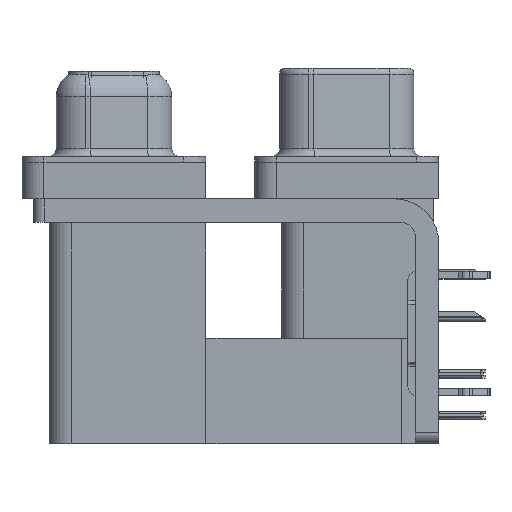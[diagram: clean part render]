
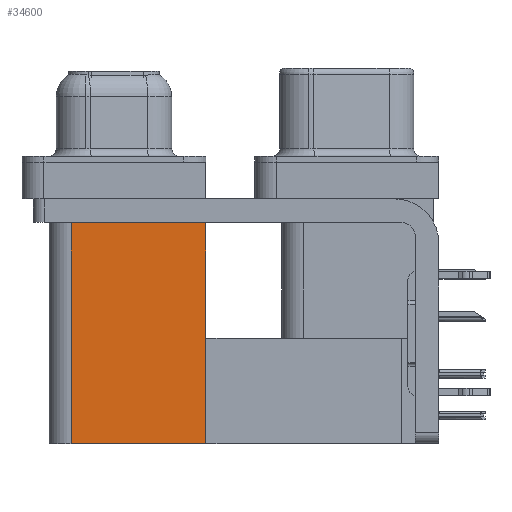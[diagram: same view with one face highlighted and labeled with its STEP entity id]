
A CAD part, left-side view. The second image highlights one B-rep face of the part: STEP entity #34600.
In plain terms, the highlighted planar face has unit normal (-1, 0, 0).
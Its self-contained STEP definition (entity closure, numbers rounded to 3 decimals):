
#1428 = VERTEX_POINT ( 'NONE', #48696 ) ;
#1985 = EDGE_CURVE ( 'NONE', #21055, #7753, #45474, .T. ) ;
#3163 = CARTESIAN_POINT ( 'NONE',  ( 3.7, 18.8, -19.2 ) ) ;
#4700 = VECTOR ( 'NONE', #24613, 1000. ) ;
#5008 = ORIENTED_EDGE ( 'NONE', *, *, #6114, .T. ) ;
#6114 = EDGE_CURVE ( 'NONE', #20795, #1428, #52254, .T. ) ;
#6152 = DIRECTION ( 'NONE',  ( 0., 0., -1. ) ) ;
#7625 = CARTESIAN_POINT ( 'NONE',  ( 3.7, 9.6, -2.5 ) ) ;
#7753 = VERTEX_POINT ( 'NONE', #36050 ) ;
#10634 = EDGE_CURVE ( 'NONE', #1428, #7753, #16259, .T. ) ;
#11768 = CARTESIAN_POINT ( 'NONE',  ( 3.7, 18.8, -19.2 ) ) ;
#14082 = DIRECTION ( 'NONE',  ( 0., 0., 1. ) ) ;
#14524 = PLANE ( 'NONE',  #26805 ) ;
#14706 = CARTESIAN_POINT ( 'NONE',  ( 3.7, 9.6, -19.2 ) ) ;
#16259 = LINE ( 'NONE', #7625, #26519 ) ;
#19075 = ORIENTED_EDGE ( 'NONE', *, *, #36004, .F. ) ;
#19764 = VECTOR ( 'NONE', #27537, 1000. ) ;
#20795 = VERTEX_POINT ( 'NONE', #32246 ) ;
#21055 = VERTEX_POINT ( 'NONE', #3163 ) ;
#23094 = VECTOR ( 'NONE', #14082, 1000. ) ;
#24613 = DIRECTION ( 'NONE',  ( 0., 0., 1. ) ) ;
#26519 = VECTOR ( 'NONE', #27983, 1000. ) ;
#26805 = AXIS2_PLACEMENT_3D ( 'NONE', #39339, #52152, #6152 ) ;
#27537 = DIRECTION ( 'NONE',  ( 0., 1., 0. ) ) ;
#27983 = DIRECTION ( 'NONE',  ( 0., 1., 0. ) ) ;
#29091 = ORIENTED_EDGE ( 'NONE', *, *, #10634, .T. ) ;
#29408 = EDGE_LOOP ( 'NONE', ( #29091, #31082, #19075, #5008 ) ) ;
#31082 = ORIENTED_EDGE ( 'NONE', *, *, #1985, .F. ) ;
#32246 = CARTESIAN_POINT ( 'NONE',  ( 3.7, 9.6, -19.2 ) ) ;
#34600 = ADVANCED_FACE ( 'NONE', ( #52696 ), #14524, .F. ) ;
#36004 = EDGE_CURVE ( 'NONE', #20795, #21055, #52892, .T. ) ;
#36050 = CARTESIAN_POINT ( 'NONE',  ( 3.7, 18.8, -2.5 ) ) ;
#39339 = CARTESIAN_POINT ( 'NONE',  ( 3.7, 9.6, -19.2 ) ) ;
#45474 = LINE ( 'NONE', #11768, #4700 ) ;
#47240 = CARTESIAN_POINT ( 'NONE',  ( 3.7, 9.6, -19.2 ) ) ;
#48696 = CARTESIAN_POINT ( 'NONE',  ( 3.7, 9.6, -2.5 ) ) ;
#52152 = DIRECTION ( 'NONE',  ( 1., 0., 0. ) ) ;
#52254 = LINE ( 'NONE', #47240, #23094 ) ;
#52696 = FACE_OUTER_BOUND ( 'NONE', #29408, .T. ) ;
#52892 = LINE ( 'NONE', #14706, #19764 ) ;
